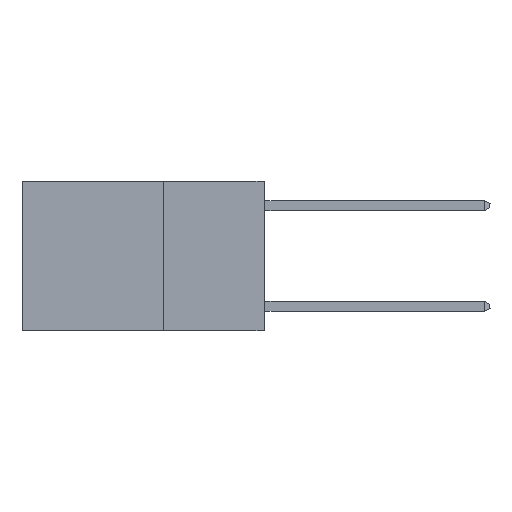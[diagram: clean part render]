
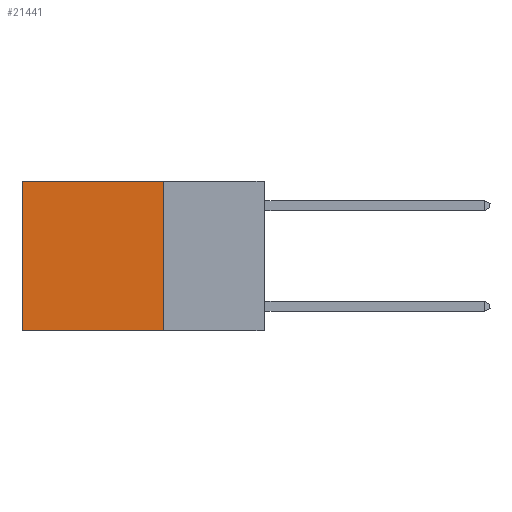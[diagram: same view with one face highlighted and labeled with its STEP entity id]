
A CAD part, left-side view. The second image highlights one B-rep face of the part: STEP entity #21441.
In plain terms, the highlighted planar face has unit normal (-1, 0, 0).
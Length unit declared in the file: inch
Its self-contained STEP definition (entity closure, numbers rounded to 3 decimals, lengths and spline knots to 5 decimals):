
#173 = EDGE_CURVE ( 'NONE', #23166, #9499, #755, .T. ) ;
#623 = DIRECTION ( 'NONE',  ( 0., 1., 0. ) ) ;
#755 = LINE ( 'NONE', #10692, #23549 ) ;
#1415 = DIRECTION ( 'NONE',  ( 0., 0., -1. ) ) ;
#2749 = CARTESIAN_POINT ( 'NONE',  ( 0.2625, 0.25, 0. ) ) ;
#2874 = PLANE ( 'NONE',  #3266 ) ;
#3266 = AXIS2_PLACEMENT_3D ( 'NONE', #2749, #10408, #8533 ) ;
#4380 = DIRECTION ( 'NONE',  ( 0., 1., 0. ) ) ;
#5656 = LINE ( 'NONE', #22751, #12551 ) ;
#6265 = LINE ( 'NONE', #21591, #21126 ) ;
#7006 = VERTEX_POINT ( 'NONE', #9960 ) ;
#7559 = EDGE_CURVE ( 'NONE', #7006, #21004, #6265, .T. ) ;
#7923 = DIRECTION ( 'NONE',  ( 0., 0., -1. ) ) ;
#8533 = DIRECTION ( 'NONE',  ( 0., 0., -1. ) ) ;
#8963 = LINE ( 'NONE', #14745, #24218 ) ;
#9499 = VERTEX_POINT ( 'NONE', #21950 ) ;
#9744 = ORIENTED_EDGE ( 'NONE', *, *, #23442, .T. ) ;
#9960 = CARTESIAN_POINT ( 'NONE',  ( 0.2625, 0.25, -0.37 ) ) ;
#10082 = EDGE_CURVE ( 'NONE', #23166, #7006, #8963, .T. ) ;
#10408 = DIRECTION ( 'NONE',  ( 1., 0., 0. ) ) ;
#10692 = CARTESIAN_POINT ( 'NONE',  ( 0.2625, 0.25, 0. ) ) ;
#11000 = EDGE_LOOP ( 'NONE', ( #9744, #22365, #14817, #18399 ) ) ;
#12551 = VECTOR ( 'NONE', #7923, 39.37008 ) ;
#14745 = CARTESIAN_POINT ( 'NONE',  ( 0.2625, 0.25, 0. ) ) ;
#14817 = ORIENTED_EDGE ( 'NONE', *, *, #10082, .F. ) ;
#18119 = CARTESIAN_POINT ( 'NONE',  ( 0.2625, 0.6, -0.37 ) ) ;
#18243 = CARTESIAN_POINT ( 'NONE',  ( 0.2625, 0.25, 0. ) ) ;
#18399 = ORIENTED_EDGE ( 'NONE', *, *, #173, .T. ) ;
#21004 = VERTEX_POINT ( 'NONE', #18119 ) ;
#21126 = VECTOR ( 'NONE', #4380, 39.37008 ) ;
#21441 = ADVANCED_FACE ( 'NONE', ( #21863 ), #2874, .F. ) ;
#21591 = CARTESIAN_POINT ( 'NONE',  ( 0.2625, 0.25, -0.37 ) ) ;
#21863 = FACE_OUTER_BOUND ( 'NONE', #11000, .T. ) ;
#21950 = CARTESIAN_POINT ( 'NONE',  ( 0.2625, 0.6, 0. ) ) ;
#22365 = ORIENTED_EDGE ( 'NONE', *, *, #7559, .F. ) ;
#22751 = CARTESIAN_POINT ( 'NONE',  ( 0.2625, 0.6, 0. ) ) ;
#23166 = VERTEX_POINT ( 'NONE', #18243 ) ;
#23442 = EDGE_CURVE ( 'NONE', #9499, #21004, #5656, .T. ) ;
#23549 = VECTOR ( 'NONE', #623, 39.37008 ) ;
#24218 = VECTOR ( 'NONE', #1415, 39.37008 ) ;
